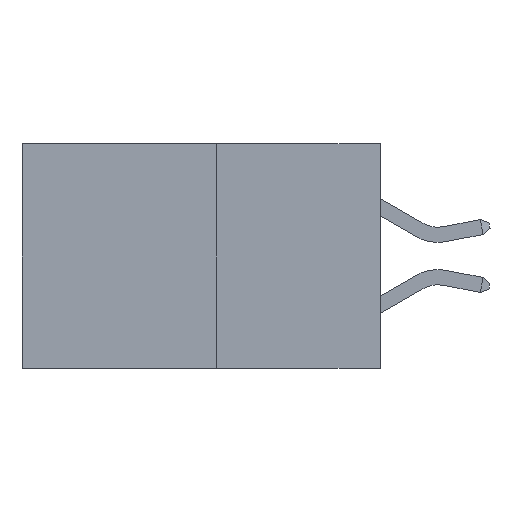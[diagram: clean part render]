
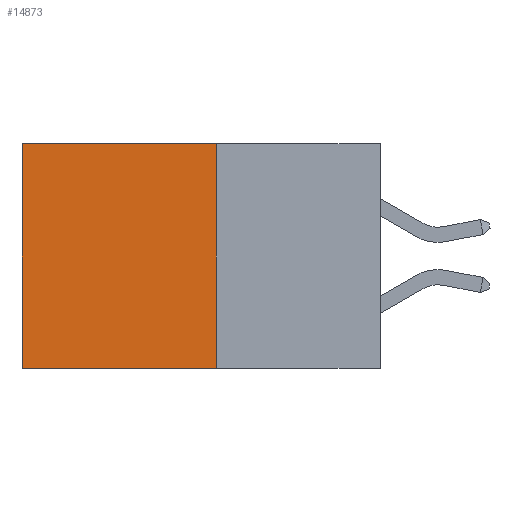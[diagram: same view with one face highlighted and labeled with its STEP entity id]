
A CAD part, left-side view. The second image highlights one B-rep face of the part: STEP entity #14873.
In plain terms, the highlighted planar face has unit normal (-1, 0, 0).
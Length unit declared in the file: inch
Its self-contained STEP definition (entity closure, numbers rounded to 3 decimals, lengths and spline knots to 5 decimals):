
#1642 = EDGE_CURVE ( 'NONE', #22368, #25346, #21827, .T. ) ;
#2514 = CARTESIAN_POINT ( 'NONE',  ( 0.277, 0.59, -0.37 ) ) ;
#3513 = VECTOR ( 'NONE', #27916, 39.37008 ) ;
#3552 = LINE ( 'NONE', #32821, #17550 ) ;
#4182 = VERTEX_POINT ( 'NONE', #2514 ) ;
#7686 = CARTESIAN_POINT ( 'NONE',  ( 0.277, 0.27, -0.37 ) ) ;
#9069 = LINE ( 'NONE', #26392, #32168 ) ;
#9572 = DIRECTION ( 'NONE',  ( 0., 0., -1. ) ) ;
#9769 = CARTESIAN_POINT ( 'NONE',  ( 0.277, 0.27, -0.37 ) ) ;
#9804 = CARTESIAN_POINT ( 'NONE',  ( 0.277, 0.27, 0. ) ) ;
#9940 = VERTEX_POINT ( 'NONE', #14105 ) ;
#12012 = CARTESIAN_POINT ( 'NONE',  ( 0.277, 0.27, -0.37 ) ) ;
#14105 = CARTESIAN_POINT ( 'NONE',  ( 0.277, 0.59, 0. ) ) ;
#14873 = ADVANCED_FACE ( 'NONE', ( #19411 ), #32765, .F. ) ;
#16263 = DIRECTION ( 'NONE',  ( 0., 1., 0. ) ) ;
#16688 = CARTESIAN_POINT ( 'NONE',  ( 0.277, 0.27, 0. ) ) ;
#16709 = AXIS2_PLACEMENT_3D ( 'NONE', #7686, #35523, #18899 ) ;
#17463 = EDGE_CURVE ( 'NONE', #22368, #9940, #18399, .T. ) ;
#17550 = VECTOR ( 'NONE', #16263, 39.37008 ) ;
#18399 = LINE ( 'NONE', #16688, #3513 ) ;
#18899 = DIRECTION ( 'NONE',  ( 0., 0., -1. ) ) ;
#19411 = FACE_OUTER_BOUND ( 'NONE', #20731, .T. ) ;
#20731 = EDGE_LOOP ( 'NONE', ( #24936, #26746, #29454, #29570 ) ) ;
#21827 = LINE ( 'NONE', #9769, #35696 ) ;
#22368 = VERTEX_POINT ( 'NONE', #9804 ) ;
#24936 = ORIENTED_EDGE ( 'NONE', *, *, #29281, .T. ) ;
#25346 = VERTEX_POINT ( 'NONE', #12012 ) ;
#26392 = CARTESIAN_POINT ( 'NONE',  ( 0.277, 0.59, -0.37 ) ) ;
#26746 = ORIENTED_EDGE ( 'NONE', *, *, #31822, .F. ) ;
#27916 = DIRECTION ( 'NONE',  ( 0., 1., 0. ) ) ;
#29182 = DIRECTION ( 'NONE',  ( 0., 0., -1. ) ) ;
#29281 = EDGE_CURVE ( 'NONE', #9940, #4182, #9069, .T. ) ;
#29454 = ORIENTED_EDGE ( 'NONE', *, *, #1642, .F. ) ;
#29570 = ORIENTED_EDGE ( 'NONE', *, *, #17463, .T. ) ;
#31822 = EDGE_CURVE ( 'NONE', #25346, #4182, #3552, .T. ) ;
#32168 = VECTOR ( 'NONE', #29182, 39.37008 ) ;
#32765 = PLANE ( 'NONE',  #16709 ) ;
#32821 = CARTESIAN_POINT ( 'NONE',  ( 0.277, 0.27, -0.37 ) ) ;
#35523 = DIRECTION ( 'NONE',  ( 1., 0., 0. ) ) ;
#35696 = VECTOR ( 'NONE', #9572, 39.37008 ) ;
